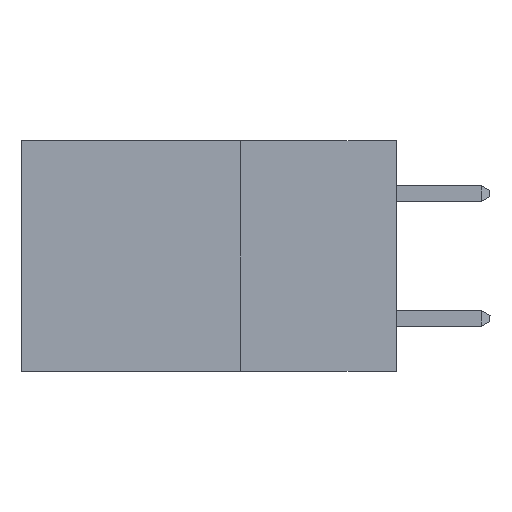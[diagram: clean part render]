
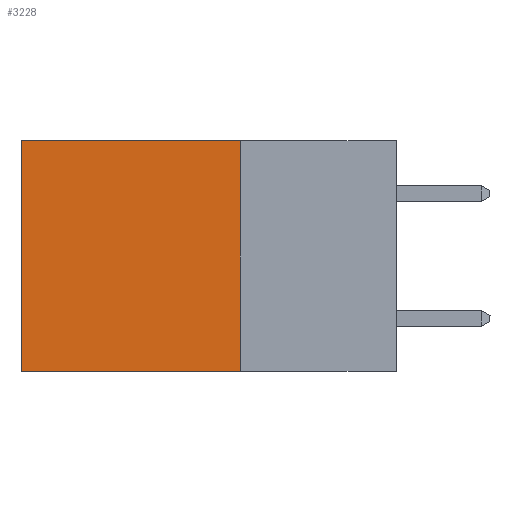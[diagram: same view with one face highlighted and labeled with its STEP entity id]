
A CAD part, left-side view. The second image highlights one B-rep face of the part: STEP entity #3228.
In plain terms, the highlighted planar face has unit normal (-1, 0, 0).
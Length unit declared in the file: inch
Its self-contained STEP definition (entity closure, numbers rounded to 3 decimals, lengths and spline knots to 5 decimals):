
#53 = EDGE_CURVE ( 'NONE', #8160, #4643, #5413, .T. ) ;
#333 = EDGE_CURVE ( 'NONE', #2726, #4643, #6923, .T. ) ;
#469 = DIRECTION ( 'NONE',  ( 0., 0., -1. ) ) ;
#851 = CARTESIAN_POINT ( 'NONE',  ( 0.2615, 0.25, -0.37 ) ) ;
#1062 = ORIENTED_EDGE ( 'NONE', *, *, #6528, .F. ) ;
#1143 = LINE ( 'NONE', #3337, #4946 ) ;
#1314 = VERTEX_POINT ( 'NONE', #8573 ) ;
#1528 = DIRECTION ( 'NONE',  ( 1., 0., 0. ) ) ;
#1694 = PLANE ( 'NONE',  #4020 ) ;
#2367 = CARTESIAN_POINT ( 'NONE',  ( 0.2615, 0.25, -0.37 ) ) ;
#2726 = VERTEX_POINT ( 'NONE', #2367 ) ;
#2732 = LINE ( 'NONE', #9004, #6389 ) ;
#3228 = ADVANCED_FACE ( 'NONE', ( #4557 ), #1694, .F. ) ;
#3238 = DIRECTION ( 'NONE',  ( 0., 0., -1. ) ) ;
#3337 = CARTESIAN_POINT ( 'NONE',  ( 0.2615, 0.25, -0.37 ) ) ;
#4020 = AXIS2_PLACEMENT_3D ( 'NONE', #4579, #1528, #469 ) ;
#4318 = EDGE_LOOP ( 'NONE', ( #5622, #6394, #1062, #4676 ) ) ;
#4557 = FACE_OUTER_BOUND ( 'NONE', #4318, .T. ) ;
#4579 = CARTESIAN_POINT ( 'NONE',  ( 0.2615, 0.25, -0.37 ) ) ;
#4643 = VERTEX_POINT ( 'NONE', #4914 ) ;
#4676 = ORIENTED_EDGE ( 'NONE', *, *, #5568, .T. ) ;
#4914 = CARTESIAN_POINT ( 'NONE',  ( 0.2615, 0.6, -0.37 ) ) ;
#4946 = VECTOR ( 'NONE', #3238, 39.37008 ) ;
#5076 = VECTOR ( 'NONE', #5482, 39.37008 ) ;
#5413 = LINE ( 'NONE', #6314, #7036 ) ;
#5482 = DIRECTION ( 'NONE',  ( 0., 1., 0. ) ) ;
#5568 = EDGE_CURVE ( 'NONE', #1314, #8160, #2732, .T. ) ;
#5622 = ORIENTED_EDGE ( 'NONE', *, *, #53, .T. ) ;
#6314 = CARTESIAN_POINT ( 'NONE',  ( 0.2615, 0.6, -0.37 ) ) ;
#6389 = VECTOR ( 'NONE', #8963, 39.37008 ) ;
#6394 = ORIENTED_EDGE ( 'NONE', *, *, #333, .F. ) ;
#6528 = EDGE_CURVE ( 'NONE', #1314, #2726, #1143, .T. ) ;
#6890 = CARTESIAN_POINT ( 'NONE',  ( 0.2615, 0.6, 0. ) ) ;
#6923 = LINE ( 'NONE', #851, #5076 ) ;
#7036 = VECTOR ( 'NONE', #7232, 39.37008 ) ;
#7232 = DIRECTION ( 'NONE',  ( 0., 0., -1. ) ) ;
#8160 = VERTEX_POINT ( 'NONE', #6890 ) ;
#8573 = CARTESIAN_POINT ( 'NONE',  ( 0.2615, 0.25, 0. ) ) ;
#8963 = DIRECTION ( 'NONE',  ( 0., 1., 0. ) ) ;
#9004 = CARTESIAN_POINT ( 'NONE',  ( 0.2615, 0.25, 0. ) ) ;
